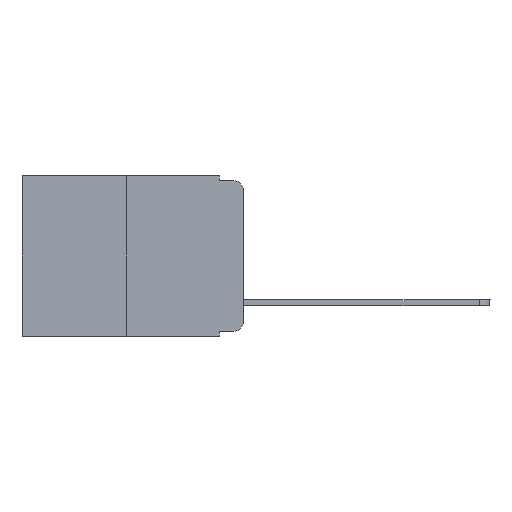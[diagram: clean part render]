
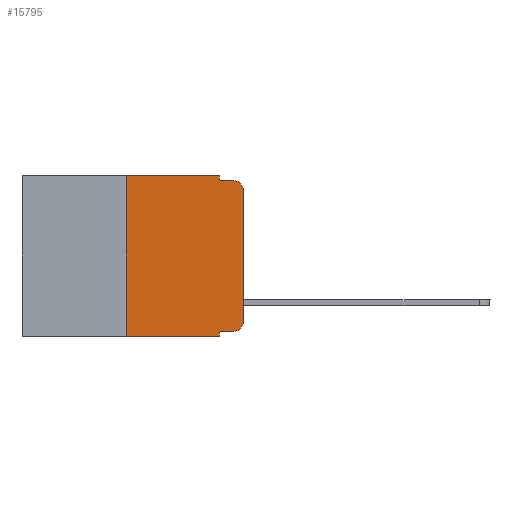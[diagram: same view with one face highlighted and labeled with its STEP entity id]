
A CAD part, left-side view. The second image highlights one B-rep face of the part: STEP entity #15795.
In plain terms, the highlighted planar face has unit normal (-1, 0, 0).
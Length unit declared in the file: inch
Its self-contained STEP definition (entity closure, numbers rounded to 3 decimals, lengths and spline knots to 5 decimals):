
#65 = CARTESIAN_POINT ( 'NONE',  ( 0., 0.051, 0. ) ) ;
#240 = CARTESIAN_POINT ( 'NONE',  ( 0., 0.02, -0.01 ) ) ;
#459 = DIRECTION ( 'NONE',  ( 0., 0., -1. ) ) ;
#1262 = EDGE_LOOP ( 'NONE', ( #2624, #4882, #10989, #20332, #9874, #14902, #9370, #3421, #11314, #12479 ) ) ;
#1426 = CARTESIAN_POINT ( 'NONE',  ( 0., 0.473, 0. ) ) ;
#1696 = VERTEX_POINT ( 'NONE', #21224 ) ;
#1805 = DIRECTION ( 'NONE',  ( 0., 0., -1. ) ) ;
#2624 = ORIENTED_EDGE ( 'NONE', *, *, #16623, .T. ) ;
#2637 = VERTEX_POINT ( 'NONE', #20696 ) ;
#3090 = EDGE_CURVE ( 'NONE', #22164, #18253, #6282, .T. ) ;
#3377 = CARTESIAN_POINT ( 'NONE',  ( 0., 0.051, -0.333 ) ) ;
#3421 = ORIENTED_EDGE ( 'NONE', *, *, #5622, .F. ) ;
#3491 = LINE ( 'NONE', #22458, #10540 ) ;
#4311 = VECTOR ( 'NONE', #18892, 39.37008 ) ;
#4391 = AXIS2_PLACEMENT_3D ( 'NONE', #1426, #20609, #12035 ) ;
#4882 = ORIENTED_EDGE ( 'NONE', *, *, #15139, .T. ) ;
#5622 = EDGE_CURVE ( 'NONE', #2637, #18253, #21682, .T. ) ;
#5634 = FACE_OUTER_BOUND ( 'NONE', #1262, .T. ) ;
#5677 = CIRCLE ( 'NONE', #15371, 0.02 ) ;
#6282 = LINE ( 'NONE', #11207, #20412 ) ;
#6938 = DIRECTION ( 'NONE',  ( 0., 0., -1. ) ) ;
#6952 = DIRECTION ( 'NONE',  ( -1., 0., 0. ) ) ;
#7250 = VECTOR ( 'NONE', #14533, 39.37008 ) ;
#7306 = VERTEX_POINT ( 'NONE', #20862 ) ;
#7606 = CARTESIAN_POINT ( 'NONE',  ( 0., 0.473, 0. ) ) ;
#8752 = EDGE_CURVE ( 'NONE', #1696, #21689, #5677, .T. ) ;
#8783 = EDGE_CURVE ( 'NONE', #13333, #12596, #20651, .T. ) ;
#9370 = ORIENTED_EDGE ( 'NONE', *, *, #3090, .T. ) ;
#9517 = EDGE_CURVE ( 'NONE', #22164, #21773, #3491, .T. ) ;
#9742 = EDGE_CURVE ( 'NONE', #21773, #13333, #15198, .T. ) ;
#9758 = LINE ( 'NONE', #12706, #14913 ) ;
#9874 = ORIENTED_EDGE ( 'NONE', *, *, #9742, .F. ) ;
#10007 = CARTESIAN_POINT ( 'NONE',  ( 0., 0.051, 0. ) ) ;
#10116 = EDGE_CURVE ( 'NONE', #12596, #16136, #9758, .T. ) ;
#10469 = CARTESIAN_POINT ( 'NONE',  ( 0., 0.051, -0.343 ) ) ;
#10540 = VECTOR ( 'NONE', #18861, 39.37008 ) ;
#10825 = VECTOR ( 'NONE', #19757, 39.37008 ) ;
#10989 = ORIENTED_EDGE ( 'NONE', *, *, #10116, .F. ) ;
#11207 = CARTESIAN_POINT ( 'NONE',  ( 0., 0.473, -0.343 ) ) ;
#11288 = DIRECTION ( 'NONE',  ( 0., -1., 0. ) ) ;
#11314 = ORIENTED_EDGE ( 'NONE', *, *, #11330, .T. ) ;
#11330 = EDGE_CURVE ( 'NONE', #2637, #1696, #20286, .T. ) ;
#12001 = CARTESIAN_POINT ( 'NONE',  ( 0., 0.051, -0.01 ) ) ;
#12035 = DIRECTION ( 'NONE',  ( 0., 0., -1. ) ) ;
#12130 = VECTOR ( 'NONE', #17108, 39.37008 ) ;
#12479 = ORIENTED_EDGE ( 'NONE', *, *, #8752, .T. ) ;
#12596 = VERTEX_POINT ( 'NONE', #12001 ) ;
#12706 = CARTESIAN_POINT ( 'NONE',  ( 0., 0.051, -0.01 ) ) ;
#13333 = VERTEX_POINT ( 'NONE', #10007 ) ;
#14203 = CARTESIAN_POINT ( 'NONE',  ( 0., 0.25, 0. ) ) ;
#14533 = DIRECTION ( 'NONE',  ( 0., 0., 1. ) ) ;
#14902 = ORIENTED_EDGE ( 'NONE', *, *, #9517, .F. ) ;
#14913 = VECTOR ( 'NONE', #21352, 39.37008 ) ;
#15139 = EDGE_CURVE ( 'NONE', #7306, #16136, #15739, .T. ) ;
#15198 = LINE ( 'NONE', #7606, #10825 ) ;
#15371 = AXIS2_PLACEMENT_3D ( 'NONE', #18997, #6952, #1805 ) ;
#15407 = LINE ( 'NONE', #15829, #7250 ) ;
#15516 = CARTESIAN_POINT ( 'NONE',  ( 0., 0., -0.313 ) ) ;
#15739 = CIRCLE ( 'NONE', #19348, 0.02 ) ;
#15795 = ADVANCED_FACE ( 'NONE', ( #5634 ), #16935, .F. ) ;
#15829 = CARTESIAN_POINT ( 'NONE',  ( 0., 0., 0. ) ) ;
#16136 = VERTEX_POINT ( 'NONE', #240 ) ;
#16147 = CARTESIAN_POINT ( 'NONE',  ( 0., 0.051, 0. ) ) ;
#16606 = CARTESIAN_POINT ( 'NONE',  ( 0., 0.25, -0.343 ) ) ;
#16623 = EDGE_CURVE ( 'NONE', #21689, #7306, #15407, .T. ) ;
#16935 = PLANE ( 'NONE',  #4391 ) ;
#17108 = DIRECTION ( 'NONE',  ( 0., -1., 0. ) ) ;
#17961 = VECTOR ( 'NONE', #459, 39.37008 ) ;
#18253 = VERTEX_POINT ( 'NONE', #10469 ) ;
#18861 = DIRECTION ( 'NONE',  ( 0., 0., 1. ) ) ;
#18892 = DIRECTION ( 'NONE',  ( 0., 0., -1. ) ) ;
#18997 = CARTESIAN_POINT ( 'NONE',  ( 0., 0.02, -0.313 ) ) ;
#19195 = DIRECTION ( 'NONE',  ( -1., 0., 0. ) ) ;
#19348 = AXIS2_PLACEMENT_3D ( 'NONE', #20764, #19195, #6938 ) ;
#19757 = DIRECTION ( 'NONE',  ( 0., -1., 0. ) ) ;
#20286 = LINE ( 'NONE', #3377, #12130 ) ;
#20332 = ORIENTED_EDGE ( 'NONE', *, *, #8783, .F. ) ;
#20412 = VECTOR ( 'NONE', #11288, 39.37008 ) ;
#20609 = DIRECTION ( 'NONE',  ( 1., 0., 0. ) ) ;
#20651 = LINE ( 'NONE', #16147, #17961 ) ;
#20696 = CARTESIAN_POINT ( 'NONE',  ( 0., 0.051, -0.333 ) ) ;
#20764 = CARTESIAN_POINT ( 'NONE',  ( 0., 0.02, -0.03 ) ) ;
#20862 = CARTESIAN_POINT ( 'NONE',  ( 0., 0., -0.03 ) ) ;
#21224 = CARTESIAN_POINT ( 'NONE',  ( 0., 0.02, -0.333 ) ) ;
#21352 = DIRECTION ( 'NONE',  ( 0., -1., 0. ) ) ;
#21682 = LINE ( 'NONE', #65, #4311 ) ;
#21689 = VERTEX_POINT ( 'NONE', #15516 ) ;
#21773 = VERTEX_POINT ( 'NONE', #14203 ) ;
#22164 = VERTEX_POINT ( 'NONE', #16606 ) ;
#22458 = CARTESIAN_POINT ( 'NONE',  ( 0., 0.25, 0. ) ) ;
